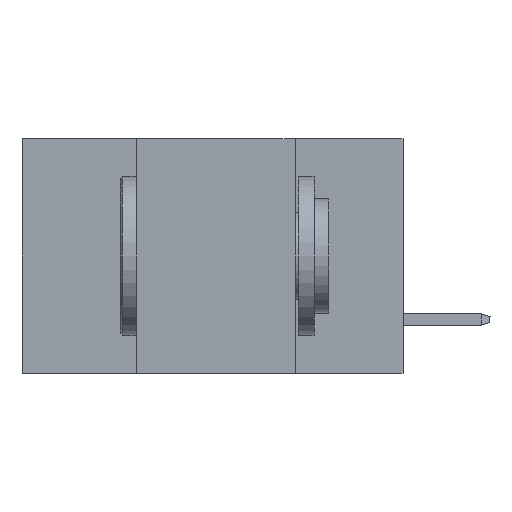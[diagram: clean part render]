
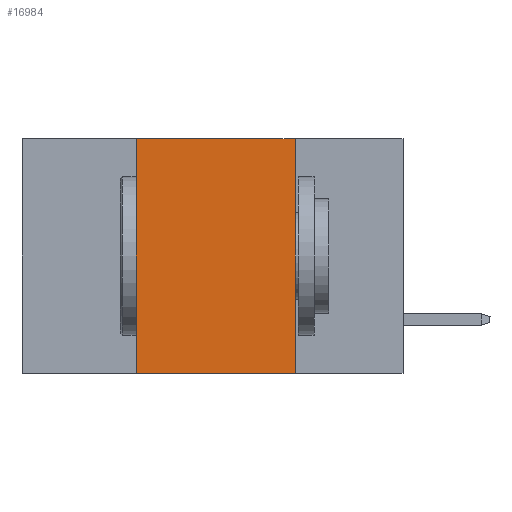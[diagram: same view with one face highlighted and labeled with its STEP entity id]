
A CAD part, left-side view. The second image highlights one B-rep face of the part: STEP entity #16984.
In plain terms, the highlighted planar face has unit normal (-1, 0, 0).
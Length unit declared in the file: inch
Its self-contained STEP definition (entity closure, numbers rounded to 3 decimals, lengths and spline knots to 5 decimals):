
#642 = CARTESIAN_POINT ( 'NONE',  ( 0., 0.42, -0.37 ) ) ;
#2236 = EDGE_LOOP ( 'NONE', ( #17577, #4157, #18338, #19161 ) ) ;
#2379 = VECTOR ( 'NONE', #8033, 39.37008 ) ;
#2930 = DIRECTION ( 'NONE',  ( 0., 0., -1. ) ) ;
#4157 = ORIENTED_EDGE ( 'NONE', *, *, #11617, .F. ) ;
#4626 = EDGE_CURVE ( 'NONE', #13290, #15941, #6669, .T. ) ;
#6476 = DIRECTION ( 'NONE',  ( 1., 0., 0. ) ) ;
#6669 = LINE ( 'NONE', #10486, #23238 ) ;
#6793 = DIRECTION ( 'NONE',  ( 0., 0., 1. ) ) ;
#8033 = DIRECTION ( 'NONE',  ( 0., -1., 0. ) ) ;
#8284 = CARTESIAN_POINT ( 'NONE',  ( 0., 0.6, 0. ) ) ;
#9059 = VECTOR ( 'NONE', #22456, 39.37008 ) ;
#10486 = CARTESIAN_POINT ( 'NONE',  ( 0., 0.42, 0. ) ) ;
#10524 = LINE ( 'NONE', #24486, #9059 ) ;
#10805 = AXIS2_PLACEMENT_3D ( 'NONE', #23875, #6476, #2930 ) ;
#11617 = EDGE_CURVE ( 'NONE', #15941, #22133, #21455, .T. ) ;
#13290 = VERTEX_POINT ( 'NONE', #642 ) ;
#13445 = EDGE_CURVE ( 'NONE', #22133, #20903, #10524, .T. ) ;
#14122 = FACE_OUTER_BOUND ( 'NONE', #2236, .T. ) ;
#15646 = VECTOR ( 'NONE', #22562, 39.37008 ) ;
#15941 = VERTEX_POINT ( 'NONE', #17367 ) ;
#15989 = LINE ( 'NONE', #23814, #15646 ) ;
#16984 = ADVANCED_FACE ( 'NONE', ( #14122 ), #19959, .F. ) ;
#17367 = CARTESIAN_POINT ( 'NONE',  ( 0., 0.42, 0. ) ) ;
#17577 = ORIENTED_EDGE ( 'NONE', *, *, #13445, .F. ) ;
#17976 = EDGE_CURVE ( 'NONE', #13290, #20903, #15989, .T. ) ;
#18338 = ORIENTED_EDGE ( 'NONE', *, *, #4626, .F. ) ;
#18767 = CARTESIAN_POINT ( 'NONE',  ( 0., 0.17, 0. ) ) ;
#18918 = CARTESIAN_POINT ( 'NONE',  ( 0., 0.17, -0.37 ) ) ;
#19161 = ORIENTED_EDGE ( 'NONE', *, *, #17976, .T. ) ;
#19959 = PLANE ( 'NONE',  #10805 ) ;
#20903 = VERTEX_POINT ( 'NONE', #18918 ) ;
#21455 = LINE ( 'NONE', #8284, #2379 ) ;
#22133 = VERTEX_POINT ( 'NONE', #18767 ) ;
#22456 = DIRECTION ( 'NONE',  ( 0., 0., -1. ) ) ;
#22562 = DIRECTION ( 'NONE',  ( 0., -1., 0. ) ) ;
#23238 = VECTOR ( 'NONE', #6793, 39.37008 ) ;
#23814 = CARTESIAN_POINT ( 'NONE',  ( 0., 0.6, -0.37 ) ) ;
#23875 = CARTESIAN_POINT ( 'NONE',  ( 0., 0.6, 0. ) ) ;
#24486 = CARTESIAN_POINT ( 'NONE',  ( 0., 0.17, 0. ) ) ;
